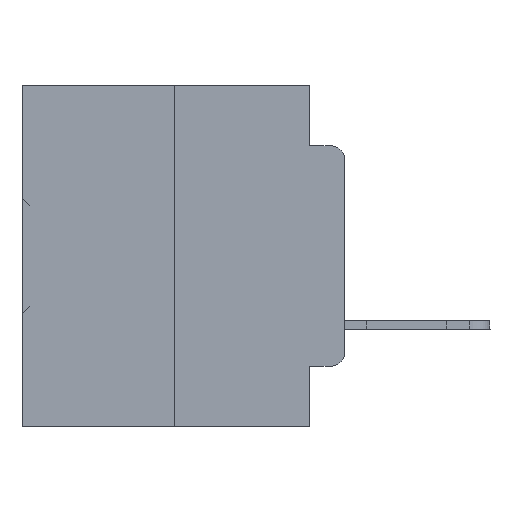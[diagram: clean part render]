
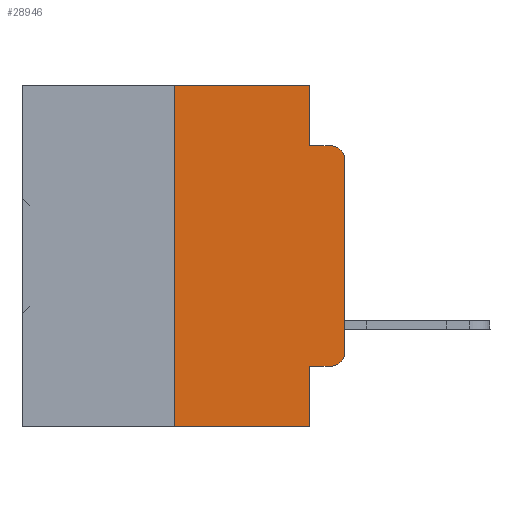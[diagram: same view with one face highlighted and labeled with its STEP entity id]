
A CAD part, left-side view. The second image highlights one B-rep face of the part: STEP entity #28946.
In plain terms, the highlighted planar face has unit normal (-1, 0, 0).
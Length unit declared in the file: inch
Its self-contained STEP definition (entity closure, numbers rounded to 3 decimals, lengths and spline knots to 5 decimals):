
#243 = CARTESIAN_POINT ( 'NONE',  ( 0., 0.473, 0. ) ) ;
#536 = LINE ( 'NONE', #31892, #23179 ) ;
#613 = FACE_OUTER_BOUND ( 'NONE', #14851, .T. ) ;
#642 = ORIENTED_EDGE ( 'NONE', *, *, #12429, .F. ) ;
#831 = EDGE_CURVE ( 'NONE', #5731, #33279, #21531, .T. ) ;
#1378 = VECTOR ( 'NONE', #20270, 39.37008 ) ;
#1449 = DIRECTION ( 'NONE',  ( 0., -1., 0. ) ) ;
#1664 = VERTEX_POINT ( 'NONE', #4735 ) ;
#1667 = VERTEX_POINT ( 'NONE', #16132 ) ;
#2015 = CARTESIAN_POINT ( 'NONE',  ( 0., 0.051, -0.0885 ) ) ;
#2356 = DIRECTION ( 'NONE',  ( 0., 0., -1. ) ) ;
#2817 = LINE ( 'NONE', #14781, #1378 ) ;
#3646 = DIRECTION ( 'NONE',  ( 1., 0., 0. ) ) ;
#4088 = CARTESIAN_POINT ( 'NONE',  ( 0., 0.473, -0.5 ) ) ;
#4735 = CARTESIAN_POINT ( 'NONE',  ( 0., 0.02, -0.4115 ) ) ;
#5650 = VECTOR ( 'NONE', #30293, 39.37008 ) ;
#5731 = VERTEX_POINT ( 'NONE', #25486 ) ;
#5881 = EDGE_CURVE ( 'NONE', #23868, #1667, #32832, .T. ) ;
#6183 = VERTEX_POINT ( 'NONE', #9604 ) ;
#7296 = ORIENTED_EDGE ( 'NONE', *, *, #17413, .F. ) ;
#7343 = AXIS2_PLACEMENT_3D ( 'NONE', #31374, #28112, #10450 ) ;
#8329 = ORIENTED_EDGE ( 'NONE', *, *, #28291, .F. ) ;
#8423 = VERTEX_POINT ( 'NONE', #9519 ) ;
#9457 = DIRECTION ( 'NONE',  ( 0., -1., 0. ) ) ;
#9519 = CARTESIAN_POINT ( 'NONE',  ( 0., 0.051, -0.0885 ) ) ;
#9604 = CARTESIAN_POINT ( 'NONE',  ( 0., 0.051, -0.4115 ) ) ;
#10209 = AXIS2_PLACEMENT_3D ( 'NONE', #243, #3646, #15225 ) ;
#10424 = CARTESIAN_POINT ( 'NONE',  ( 0., 0.051, 0. ) ) ;
#10450 = DIRECTION ( 'NONE',  ( 0., 0., -1. ) ) ;
#11810 = PLANE ( 'NONE',  #10209 ) ;
#12095 = VERTEX_POINT ( 'NONE', #17121 ) ;
#12429 = EDGE_CURVE ( 'NONE', #6183, #33279, #18601, .T. ) ;
#12520 = CARTESIAN_POINT ( 'NONE',  ( 0., 0.25, 0. ) ) ;
#12622 = DIRECTION ( 'NONE',  ( 0., -1., 0. ) ) ;
#12961 = CARTESIAN_POINT ( 'NONE',  ( 0., 0.02, -0.0885 ) ) ;
#14278 = VECTOR ( 'NONE', #12622, 39.37008 ) ;
#14781 = CARTESIAN_POINT ( 'NONE',  ( 0., 0., 0. ) ) ;
#14851 = EDGE_LOOP ( 'NONE', ( #32273, #32213, #8329, #27612, #26689, #7296, #23038, #642, #22015, #19993 ) ) ;
#15225 = DIRECTION ( 'NONE',  ( 0., 0., -1. ) ) ;
#15404 = CARTESIAN_POINT ( 'NONE',  ( 0., 0.051, -0.5 ) ) ;
#15528 = EDGE_CURVE ( 'NONE', #1664, #12095, #20685, .T. ) ;
#15646 = DIRECTION ( 'NONE',  ( -1., 0., 0. ) ) ;
#16132 = CARTESIAN_POINT ( 'NONE',  ( 0., 0.051, 0. ) ) ;
#16168 = AXIS2_PLACEMENT_3D ( 'NONE', #33107, #15646, #18669 ) ;
#16822 = EDGE_CURVE ( 'NONE', #6183, #1664, #25123, .T. ) ;
#16856 = CIRCLE ( 'NONE', #16168, 0.02 ) ;
#17121 = CARTESIAN_POINT ( 'NONE',  ( 0., 0., -0.3915 ) ) ;
#17150 = CARTESIAN_POINT ( 'NONE',  ( 0., 0.051, 0. ) ) ;
#17371 = EDGE_CURVE ( 'NONE', #12095, #35885, #2817, .T. ) ;
#17413 = EDGE_CURVE ( 'NONE', #5731, #23868, #536, .T. ) ;
#18601 = LINE ( 'NONE', #10424, #33683 ) ;
#18669 = DIRECTION ( 'NONE',  ( 0., 0., -1. ) ) ;
#19993 = ORIENTED_EDGE ( 'NONE', *, *, #15528, .T. ) ;
#20270 = DIRECTION ( 'NONE',  ( 0., 0., 1. ) ) ;
#20685 = CIRCLE ( 'NONE', #7343, 0.02 ) ;
#21531 = LINE ( 'NONE', #4088, #14278 ) ;
#21632 = EDGE_CURVE ( 'NONE', #1667, #8423, #36928, .T. ) ;
#22015 = ORIENTED_EDGE ( 'NONE', *, *, #16822, .T. ) ;
#23038 = ORIENTED_EDGE ( 'NONE', *, *, #831, .T. ) ;
#23179 = VECTOR ( 'NONE', #23492, 39.37008 ) ;
#23492 = DIRECTION ( 'NONE',  ( 0., 0., 1. ) ) ;
#23868 = VERTEX_POINT ( 'NONE', #12520 ) ;
#23886 = CARTESIAN_POINT ( 'NONE',  ( 0., 0.473, 0. ) ) ;
#25005 = VECTOR ( 'NONE', #9457, 39.37008 ) ;
#25110 = CARTESIAN_POINT ( 'NONE',  ( 0., 0., -0.1085 ) ) ;
#25123 = LINE ( 'NONE', #30475, #5650 ) ;
#25486 = CARTESIAN_POINT ( 'NONE',  ( 0., 0.25, -0.5 ) ) ;
#26689 = ORIENTED_EDGE ( 'NONE', *, *, #5881, .F. ) ;
#27365 = VERTEX_POINT ( 'NONE', #12961 ) ;
#27612 = ORIENTED_EDGE ( 'NONE', *, *, #21632, .F. ) ;
#28015 = LINE ( 'NONE', #2015, #35083 ) ;
#28112 = DIRECTION ( 'NONE',  ( -1., 0., 0. ) ) ;
#28291 = EDGE_CURVE ( 'NONE', #8423, #27365, #28015, .T. ) ;
#28946 = ADVANCED_FACE ( 'NONE', ( #613 ), #11810, .F. ) ;
#30293 = DIRECTION ( 'NONE',  ( 0., -1., 0. ) ) ;
#30475 = CARTESIAN_POINT ( 'NONE',  ( 0., 0.051, -0.4115 ) ) ;
#31123 = VECTOR ( 'NONE', #2356, 39.37008 ) ;
#31374 = CARTESIAN_POINT ( 'NONE',  ( 0., 0.02, -0.3915 ) ) ;
#31892 = CARTESIAN_POINT ( 'NONE',  ( 0., 0.25, 0. ) ) ;
#32213 = ORIENTED_EDGE ( 'NONE', *, *, #34631, .T. ) ;
#32273 = ORIENTED_EDGE ( 'NONE', *, *, #17371, .T. ) ;
#32832 = LINE ( 'NONE', #23886, #25005 ) ;
#33107 = CARTESIAN_POINT ( 'NONE',  ( 0., 0.02, -0.1085 ) ) ;
#33279 = VERTEX_POINT ( 'NONE', #15404 ) ;
#33683 = VECTOR ( 'NONE', #36466, 39.37008 ) ;
#34631 = EDGE_CURVE ( 'NONE', #35885, #27365, #16856, .T. ) ;
#35083 = VECTOR ( 'NONE', #1449, 39.37008 ) ;
#35885 = VERTEX_POINT ( 'NONE', #25110 ) ;
#36466 = DIRECTION ( 'NONE',  ( 0., 0., -1. ) ) ;
#36928 = LINE ( 'NONE', #17150, #31123 ) ;
